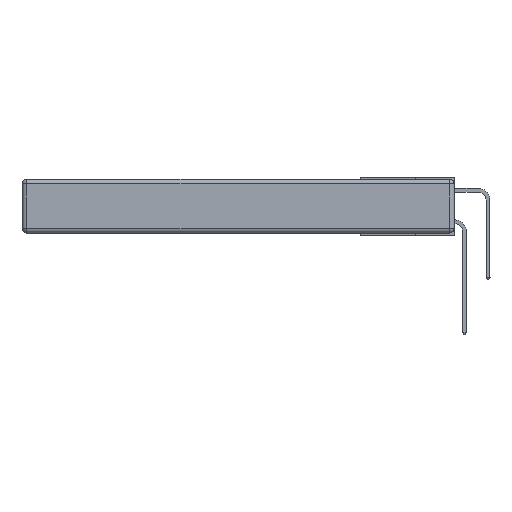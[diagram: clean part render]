
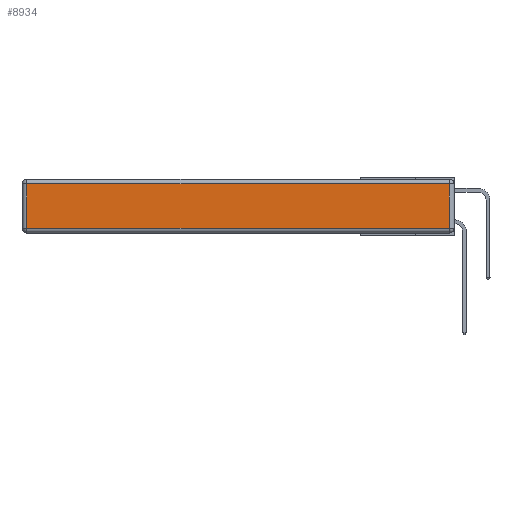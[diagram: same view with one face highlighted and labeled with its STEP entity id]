
A CAD part, left-side view. The second image highlights one B-rep face of the part: STEP entity #8934.
In plain terms, the highlighted planar face has unit normal (-1, 0, 0).
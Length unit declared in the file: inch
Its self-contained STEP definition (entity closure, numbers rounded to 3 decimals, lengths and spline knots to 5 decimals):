
#426 = CARTESIAN_POINT ( 'NONE',  ( 0., 0.03, -0.313 ) ) ;
#3254 = VERTEX_POINT ( 'NONE', #426 ) ;
#4617 = EDGE_CURVE ( 'NONE', #3254, #9492, #14099, .T. ) ;
#6239 = CARTESIAN_POINT ( 'NONE',  ( 0., 0., -0.313 ) ) ;
#6933 = EDGE_CURVE ( 'NONE', #37484, #19098, #32424, .T. ) ;
#7157 = DIRECTION ( 'NONE',  ( -1., 0., 0. ) ) ;
#8934 = ADVANCED_FACE ( 'NONE', ( #36465 ), #27317, .T. ) ;
#9492 = VERTEX_POINT ( 'NONE', #37457 ) ;
#11291 = EDGE_CURVE ( 'NONE', #9492, #37484, #26430, .T. ) ;
#11776 = VECTOR ( 'NONE', #12270, 39.37008 ) ;
#12270 = DIRECTION ( 'NONE',  ( 0., 1., 0. ) ) ;
#12444 = ORIENTED_EDGE ( 'NONE', *, *, #34090, .T. ) ;
#14099 = LINE ( 'NONE', #33709, #16375 ) ;
#15419 = DIRECTION ( 'NONE',  ( 0., 0., -1. ) ) ;
#16375 = VECTOR ( 'NONE', #24790, 39.37008 ) ;
#17342 = LINE ( 'NONE', #6239, #36554 ) ;
#18104 = CARTESIAN_POINT ( 'NONE',  ( 0., 2.72, -0.343 ) ) ;
#18235 = CARTESIAN_POINT ( 'NONE',  ( 0., 2.75, -0.03 ) ) ;
#18879 = DIRECTION ( 'NONE',  ( 0., 0., 1. ) ) ;
#19098 = VERTEX_POINT ( 'NONE', #19442 ) ;
#19442 = CARTESIAN_POINT ( 'NONE',  ( 0., 2.72, -0.313 ) ) ;
#22030 = ORIENTED_EDGE ( 'NONE', *, *, #6933, .T. ) ;
#23116 = CARTESIAN_POINT ( 'NONE',  ( 0., 2.72, -0.03 ) ) ;
#23316 = ORIENTED_EDGE ( 'NONE', *, *, #4617, .T. ) ;
#24790 = DIRECTION ( 'NONE',  ( 0., 0., 1. ) ) ;
#26403 = DIRECTION ( 'NONE',  ( 0., -1., 0. ) ) ;
#26430 = LINE ( 'NONE', #18235, #11776 ) ;
#27317 = PLANE ( 'NONE',  #34829 ) ;
#30608 = VECTOR ( 'NONE', #15419, 39.37008 ) ;
#32424 = LINE ( 'NONE', #18104, #30608 ) ;
#33651 = EDGE_LOOP ( 'NONE', ( #12444, #23316, #33759, #22030 ) ) ;
#33709 = CARTESIAN_POINT ( 'NONE',  ( 0., 0.03, -0.343 ) ) ;
#33759 = ORIENTED_EDGE ( 'NONE', *, *, #11291, .T. ) ;
#34090 = EDGE_CURVE ( 'NONE', #19098, #3254, #17342, .T. ) ;
#34829 = AXIS2_PLACEMENT_3D ( 'NONE', #36391, #7157, #18879 ) ;
#36391 = CARTESIAN_POINT ( 'NONE',  ( 0., 0., -0.343 ) ) ;
#36465 = FACE_OUTER_BOUND ( 'NONE', #33651, .T. ) ;
#36554 = VECTOR ( 'NONE', #26403, 39.37008 ) ;
#37457 = CARTESIAN_POINT ( 'NONE',  ( 0., 0.03, -0.03 ) ) ;
#37484 = VERTEX_POINT ( 'NONE', #23116 ) ;
